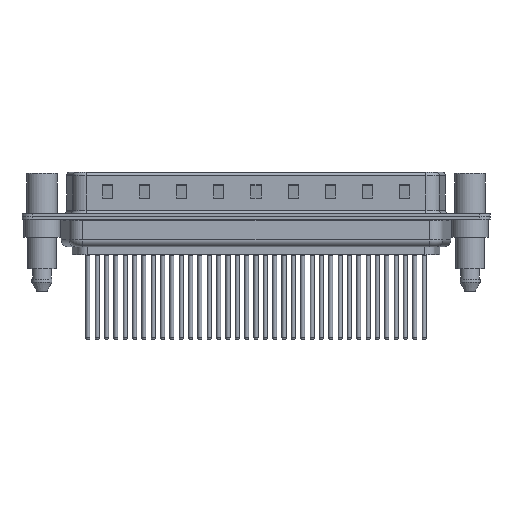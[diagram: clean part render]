
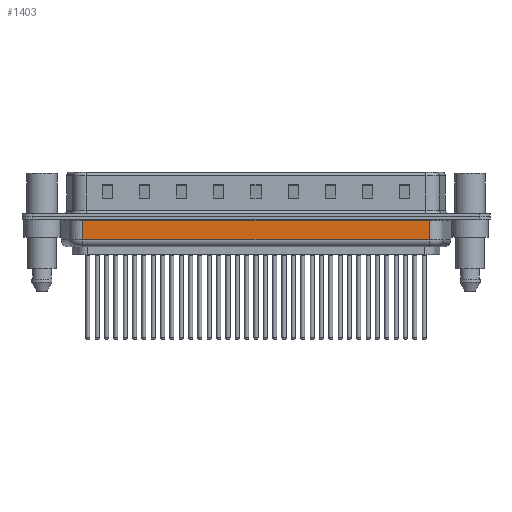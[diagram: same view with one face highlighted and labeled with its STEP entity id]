
A CAD part, front view. The second image highlights one B-rep face of the part: STEP entity #1403.
In plain terms, the highlighted planar face has unit normal (0, -1, 0).
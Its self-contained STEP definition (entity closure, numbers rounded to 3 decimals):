
#389 = VECTOR ( 'NONE', #7765, 1000. ) ;
#820 = VECTOR ( 'NONE', #20952, 1000. ) ;
#923 = LINE ( 'NONE', #18574, #9809 ) ;
#1403 = ADVANCED_FACE ( 'NONE', ( #25239 ), #13016, .F. ) ;
#1424 = DIRECTION ( 'NONE',  ( 0., 1., 0. ) ) ;
#5200 = VERTEX_POINT ( 'NONE', #18690 ) ;
#5977 = VECTOR ( 'NONE', #15134, 1000. ) ;
#7286 = LINE ( 'NONE', #16952, #5977 ) ;
#7294 = EDGE_CURVE ( 'NONE', #24424, #5200, #923, .T. ) ;
#7765 = DIRECTION ( 'NONE',  ( 1., 0., 0. ) ) ;
#8793 = DIRECTION ( 'NONE',  ( -1., 0., 0. ) ) ;
#9549 = DIRECTION ( 'NONE',  ( -1., 0., 0. ) ) ;
#9809 = VECTOR ( 'NONE', #8793, 1000. ) ;
#10163 = EDGE_LOOP ( 'NONE', ( #19006, #18936, #14891, #20276 ) ) ;
#10267 = VERTEX_POINT ( 'NONE', #15588 ) ;
#11347 = CARTESIAN_POINT ( 'NONE',  ( 6.031, -5.35, -4.5 ) ) ;
#13016 = PLANE ( 'NONE',  #14406 ) ;
#14406 = AXIS2_PLACEMENT_3D ( 'NONE', #11347, #1424, #9549 ) ;
#14891 = ORIENTED_EDGE ( 'NONE', *, *, #21429, .T. ) ;
#15008 = EDGE_CURVE ( 'NONE', #18617, #5200, #16980, .T. ) ;
#15134 = DIRECTION ( 'NONE',  ( 0., 0., 1. ) ) ;
#15393 = CARTESIAN_POINT ( 'NONE',  ( 57.469, -5.35, -0.65 ) ) ;
#15588 = CARTESIAN_POINT ( 'NONE',  ( 57.469, -5.35, -3.5 ) ) ;
#16952 = CARTESIAN_POINT ( 'NONE',  ( 57.469, -5.35, -4.5 ) ) ;
#16980 = LINE ( 'NONE', #24826, #820 ) ;
#17687 = LINE ( 'NONE', #19497, #389 ) ;
#18574 = CARTESIAN_POINT ( 'NONE',  ( 6.031, -5.35, -0.65 ) ) ;
#18617 = VERTEX_POINT ( 'NONE', #21668 ) ;
#18690 = CARTESIAN_POINT ( 'NONE',  ( 6.031, -5.35, -0.65 ) ) ;
#18936 = ORIENTED_EDGE ( 'NONE', *, *, #23395, .T. ) ;
#19006 = ORIENTED_EDGE ( 'NONE', *, *, #15008, .F. ) ;
#19497 = CARTESIAN_POINT ( 'NONE',  ( 6.031, -5.35, -3.5 ) ) ;
#20276 = ORIENTED_EDGE ( 'NONE', *, *, #7294, .T. ) ;
#20952 = DIRECTION ( 'NONE',  ( 0., 0., 1. ) ) ;
#21429 = EDGE_CURVE ( 'NONE', #10267, #24424, #7286, .T. ) ;
#21668 = CARTESIAN_POINT ( 'NONE',  ( 6.031, -5.35, -3.5 ) ) ;
#23395 = EDGE_CURVE ( 'NONE', #18617, #10267, #17687, .T. ) ;
#24424 = VERTEX_POINT ( 'NONE', #15393 ) ;
#24826 = CARTESIAN_POINT ( 'NONE',  ( 6.031, -5.35, -4.5 ) ) ;
#25239 = FACE_OUTER_BOUND ( 'NONE', #10163, .T. ) ;
